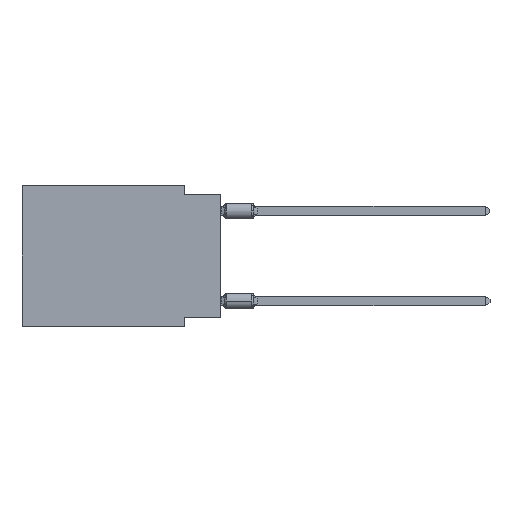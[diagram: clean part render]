
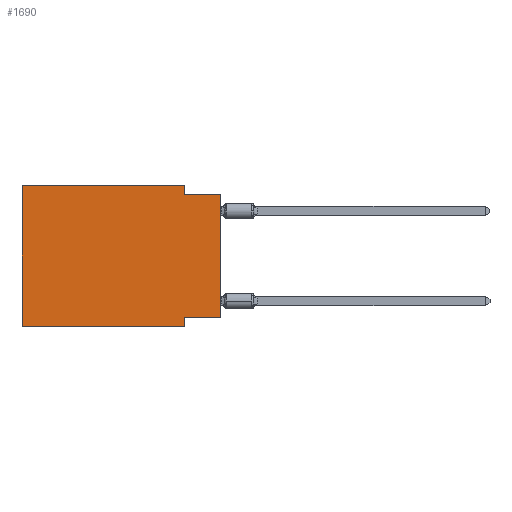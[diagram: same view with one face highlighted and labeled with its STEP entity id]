
A CAD part, left-side view. The second image highlights one B-rep face of the part: STEP entity #1690.
In plain terms, the highlighted planar face has unit normal (-1, 0, 0).
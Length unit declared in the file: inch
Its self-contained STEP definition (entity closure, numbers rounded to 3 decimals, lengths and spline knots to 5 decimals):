
#252 = LINE ( 'NONE', #17746, #14279 ) ;
#511 = VERTEX_POINT ( 'NONE', #11722 ) ;
#753 = VERTEX_POINT ( 'NONE', #15147 ) ;
#1130 = VECTOR ( 'NONE', #21214, 39.37008 ) ;
#1395 = VECTOR ( 'NONE', #7858, 39.37008 ) ;
#1690 = ADVANCED_FACE ( 'NONE', ( #2334 ), #17966, .F. ) ;
#2027 = VERTEX_POINT ( 'NONE', #10462 ) ;
#2334 = FACE_OUTER_BOUND ( 'NONE', #17868, .T. ) ;
#2755 = CARTESIAN_POINT ( 'NONE',  ( 0., 0.55, 0. ) ) ;
#2840 = EDGE_CURVE ( 'NONE', #15499, #511, #25532, .T. ) ;
#4473 = VECTOR ( 'NONE', #23220, 39.37008 ) ;
#4613 = DIRECTION ( 'NONE',  ( 1., 0., 0. ) ) ;
#5000 = VECTOR ( 'NONE', #18242, 39.37008 ) ;
#5497 = DIRECTION ( 'NONE',  ( 0., 0., 1. ) ) ;
#5569 = CARTESIAN_POINT ( 'NONE',  ( 0., 0., 0. ) ) ;
#5954 = CARTESIAN_POINT ( 'NONE',  ( 0., 0.1, 0. ) ) ;
#6389 = ORIENTED_EDGE ( 'NONE', *, *, #10185, .T. ) ;
#6778 = EDGE_CURVE ( 'NONE', #15219, #511, #20000, .T. ) ;
#7858 = DIRECTION ( 'NONE',  ( 0., 0., 1. ) ) ;
#8514 = CARTESIAN_POINT ( 'NONE',  ( 0., 0.1, -0.39 ) ) ;
#10185 = EDGE_CURVE ( 'NONE', #2027, #753, #25825, .T. ) ;
#10462 = CARTESIAN_POINT ( 'NONE',  ( 0., 0., -0.365 ) ) ;
#10511 = VERTEX_POINT ( 'NONE', #5954 ) ;
#11722 = CARTESIAN_POINT ( 'NONE',  ( 0., 0.1, -0.39 ) ) ;
#11923 = CARTESIAN_POINT ( 'NONE',  ( 0., 0., -0.365 ) ) ;
#12325 = EDGE_CURVE ( 'NONE', #15499, #17544, #25763, .T. ) ;
#12760 = EDGE_CURVE ( 'NONE', #24665, #753, #252, .T. ) ;
#12858 = VECTOR ( 'NONE', #5497, 39.37008 ) ;
#14279 = VECTOR ( 'NONE', #28392, 39.37008 ) ;
#14304 = CARTESIAN_POINT ( 'NONE',  ( 0., 0.55, 0. ) ) ;
#15147 = CARTESIAN_POINT ( 'NONE',  ( 0., 0., -0.025 ) ) ;
#15203 = EDGE_CURVE ( 'NONE', #10511, #24665, #25810, .T. ) ;
#15219 = VERTEX_POINT ( 'NONE', #17034 ) ;
#15499 = VERTEX_POINT ( 'NONE', #22462 ) ;
#16016 = CARTESIAN_POINT ( 'NONE',  ( 0., 0.1, -0.025 ) ) ;
#16514 = EDGE_CURVE ( 'NONE', #2027, #15219, #25285, .T. ) ;
#16619 = CARTESIAN_POINT ( 'NONE',  ( 0., 0.55, -0.39 ) ) ;
#17034 = CARTESIAN_POINT ( 'NONE',  ( 0., 0.1, -0.365 ) ) ;
#17224 = EDGE_CURVE ( 'NONE', #17544, #10511, #27185, .T. ) ;
#17544 = VERTEX_POINT ( 'NONE', #14304 ) ;
#17548 = DIRECTION ( 'NONE',  ( 0., 0., -1. ) ) ;
#17746 = CARTESIAN_POINT ( 'NONE',  ( 0., 0., -0.025 ) ) ;
#17868 = EDGE_LOOP ( 'NONE', ( #6389, #18414, #19481, #24456, #27880, #26887, #25959, #20801 ) ) ;
#17966 = PLANE ( 'NONE',  #18111 ) ;
#18111 = AXIS2_PLACEMENT_3D ( 'NONE', #19849, #4613, #17548 ) ;
#18242 = DIRECTION ( 'NONE',  ( 0., -1., 0. ) ) ;
#18414 = ORIENTED_EDGE ( 'NONE', *, *, #12760, .F. ) ;
#19175 = CARTESIAN_POINT ( 'NONE',  ( 0., 0.1, 0. ) ) ;
#19481 = ORIENTED_EDGE ( 'NONE', *, *, #15203, .F. ) ;
#19658 = VECTOR ( 'NONE', #25563, 39.37008 ) ;
#19849 = CARTESIAN_POINT ( 'NONE',  ( 0., 0.55, 0. ) ) ;
#20000 = LINE ( 'NONE', #8514, #22849 ) ;
#20801 = ORIENTED_EDGE ( 'NONE', *, *, #16514, .F. ) ;
#21214 = DIRECTION ( 'NONE',  ( 0., -1., 0. ) ) ;
#22462 = CARTESIAN_POINT ( 'NONE',  ( 0., 0.55, -0.39 ) ) ;
#22849 = VECTOR ( 'NONE', #24478, 39.37008 ) ;
#23220 = DIRECTION ( 'NONE',  ( 0., 0., -1. ) ) ;
#24456 = ORIENTED_EDGE ( 'NONE', *, *, #17224, .F. ) ;
#24478 = DIRECTION ( 'NONE',  ( 0., 0., -1. ) ) ;
#24665 = VERTEX_POINT ( 'NONE', #16016 ) ;
#25285 = LINE ( 'NONE', #11923, #19658 ) ;
#25338 = CARTESIAN_POINT ( 'NONE',  ( 0., 0.55, 0. ) ) ;
#25532 = LINE ( 'NONE', #16619, #1130 ) ;
#25563 = DIRECTION ( 'NONE',  ( 0., 1., 0. ) ) ;
#25763 = LINE ( 'NONE', #25338, #12858 ) ;
#25810 = LINE ( 'NONE', #19175, #4473 ) ;
#25825 = LINE ( 'NONE', #5569, #1395 ) ;
#25959 = ORIENTED_EDGE ( 'NONE', *, *, #6778, .F. ) ;
#26887 = ORIENTED_EDGE ( 'NONE', *, *, #2840, .T. ) ;
#27185 = LINE ( 'NONE', #2755, #5000 ) ;
#27880 = ORIENTED_EDGE ( 'NONE', *, *, #12325, .F. ) ;
#28392 = DIRECTION ( 'NONE',  ( 0., -1., 0. ) ) ;
